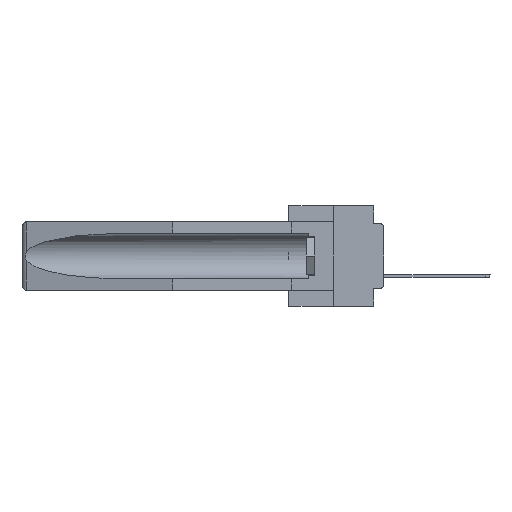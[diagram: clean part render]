
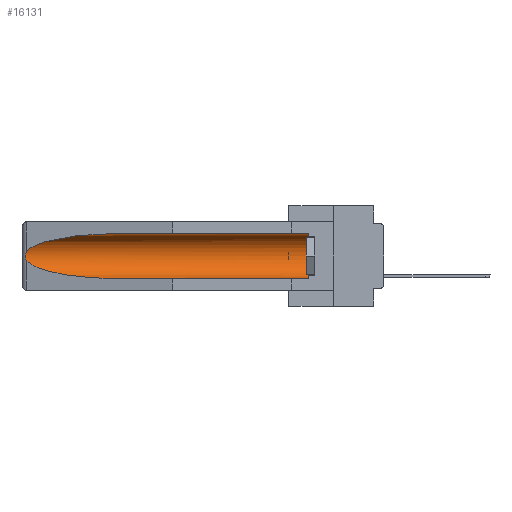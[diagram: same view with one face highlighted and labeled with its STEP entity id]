
A CAD part, left-side view. The second image highlights one B-rep face of the part: STEP entity #16131.
In plain terms, the highlighted cylindrical face has radius 2.857 mm (diameter 5.715 mm), a partial arc.
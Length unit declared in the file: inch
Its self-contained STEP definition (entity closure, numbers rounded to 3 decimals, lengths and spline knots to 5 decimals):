
#468 = CARTESIAN_POINT ( 'NONE',  ( 0.26537, 1.52718, -0.14972 ) ) ;
#720 = EDGE_CURVE ( 'NONE', #23461, #37545, #6997, .T. ) ;
#1621 = CARTESIAN_POINT ( 'NONE',  ( 0.2673, 1.53269, -0.17917 ) ) ;
#3611 = CIRCLE ( 'NONE', #32259, 0.1125 ) ;
#3714 = CYLINDRICAL_SURFACE ( 'NONE', #25135, 0.1125 ) ;
#4158 = FACE_OUTER_BOUND ( 'NONE', #36566, .T. ) ;
#4191 = CARTESIAN_POINT ( 'NONE',  ( 0.2675, 1.53308, -0.16763 ) ) ;
#4538 = VECTOR ( 'NONE', #9666, 39.37008 ) ;
#4730 = CARTESIAN_POINT ( 'NONE',  ( 0.26597, 1.5296, -0.19026 ) ) ;
#4777 = CARTESIAN_POINT ( 'NONE',  ( 0.155, -0.30754, -0.1715 ) ) ;
#5171 = EDGE_CURVE ( 'NONE', #23461, #20701, #3611, .T. ) ;
#5293 = DIRECTION ( 'NONE',  ( 0., 1., 0. ) ) ;
#6997 = LINE ( 'NONE', #7758, #8946 ) ;
#7758 = CARTESIAN_POINT ( 'NONE',  ( 0.155, -0.30754, -0.284 ) ) ;
#8514 = DIRECTION ( 'NONE',  ( 0., 0., 1. ) ) ;
#8946 = VECTOR ( 'NONE', #29276, 39.37008 ) ;
#8995 = DIRECTION ( 'NONE',  ( 0., 0., 1. ) ) ;
#9666 = DIRECTION ( 'NONE',  ( 0., 1., 0. ) ) ;
#11897 = EDGE_CURVE ( 'NONE', #32058, #24717, #37522, .T. ) ;
#11939 = CARTESIAN_POINT ( 'NONE',  ( 0.25451, 1.48313, -0.09465 ) ) ;
#12513 = VERTEX_POINT ( 'NONE', #27570 ) ;
#13298 = CARTESIAN_POINT ( 'NONE',  ( 0.26654, 1.53092, -0.15636 ) ) ;
#13831 = CARTESIAN_POINT ( 'NONE',  ( 0.2673, 1.5327, -0.16383 ) ) ;
#15137 = ORIENTED_EDGE ( 'NONE', *, *, #34715, .T. ) ;
#15309 = CARTESIAN_POINT ( 'NONE',  ( 0.155, -0.30754, -0.059 ) ) ;
#16131 = ADVANCED_FACE ( 'NONE', ( #4158 ), #3714, .F. ) ;
#16819 = CARTESIAN_POINT ( 'NONE',  ( 0.26537, 1.52718, -0.14972 ) ) ;
#18142 = CARTESIAN_POINT ( 'NONE',  ( 0.26537, 1.52718, -0.14972 ) ) ;
#18257 = CARTESIAN_POINT ( 'NONE',  ( 0.155, 0.126, -0.284 ) ) ;
#18539 = CARTESIAN_POINT ( 'NONE',  ( 0.25451, 1.48313, -0.24835 ) ) ;
#18701 = ORIENTED_EDGE ( 'NONE', *, *, #11897, .T. ) ;
#19515 = CARTESIAN_POINT ( 'NONE',  ( 0.26597, 1.52961, -0.15275 ) ) ;
#20701 = VERTEX_POINT ( 'NONE', #30123 ) ;
#23461 = VERTEX_POINT ( 'NONE', #18257 ) ;
#23571 = CARTESIAN_POINT ( 'NONE',  ( 0.155, 1.07973, -0.284 ) ) ;
#24481 = DIRECTION ( 'NONE',  ( 0., -1., 0. ) ) ;
#24717 = VERTEX_POINT ( 'NONE', #468 ) ;
#25042 = CARTESIAN_POINT ( 'NONE',  ( 0.26537, 1.52718, -0.19328 ) ) ;
#25135 = AXIS2_PLACEMENT_3D ( 'NONE', #4777, #5293, #8514 ) ;
#26280 = CARTESIAN_POINT ( 'NONE',  ( 0.26537, 1.52718, -0.19328 ) ) ;
#27570 = CARTESIAN_POINT ( 'NONE',  ( 0.26537, 1.52718, -0.19328 ) ) ;
#27589 = CARTESIAN_POINT ( 'NONE',  ( 0.21114, 1.30732, -0.284 ) ) ;
#29276 = DIRECTION ( 'NONE',  ( 0., 1., 0. ) ) ;
#30123 = CARTESIAN_POINT ( 'NONE',  ( 0.155, 0.126, -0.059 ) ) ;
#30777 = ORIENTED_EDGE ( 'NONE', *, *, #5171, .T. ) ;
#31809 = ORIENTED_EDGE ( 'NONE', *, *, #34392, .T. ) ;
#32015 = CARTESIAN_POINT ( 'NONE',  ( 0.26655, 1.53094, -0.18657 ) ) ;
#32058 = VERTEX_POINT ( 'NONE', #32993 ) ;
#32115 =( BOUNDED_CURVE ( )  B_SPLINE_CURVE ( 3, ( #25042, #18539, #27589, #36830 ),
 .UNSPECIFIED., .F., .T. ) 
 B_SPLINE_CURVE_WITH_KNOTS ( ( 4, 4 ),
 ( 0.1948, 1.5708 ),
 .UNSPECIFIED. ) 
 CURVE ( )  GEOMETRIC_REPRESENTATION_ITEM ( )  RATIONAL_B_SPLINE_CURVE ( ( 1., 0.848, 0.848, 1. ) ) 
 REPRESENTATION_ITEM ( '' )  );
#32259 = AXIS2_PLACEMENT_3D ( 'NONE', #39631, #24481, #8995 ) ;
#32327 = ORIENTED_EDGE ( 'NONE', *, *, #720, .F. ) ;
#32993 = CARTESIAN_POINT ( 'NONE',  ( 0.155, 1.07973, -0.059 ) ) ;
#33305 = EDGE_CURVE ( 'NONE', #20701, #32058, #38188, .T. ) ;
#33340 = B_SPLINE_CURVE_WITH_KNOTS ( 'NONE', 3,
 ( #16819, #19515, #13298, #13831, #4191, #38449, #1621, #32015, #4730, #26280 ),
 .UNSPECIFIED., .F., .F.,
 ( 4, 2, 2, 2, 4 ),
 ( 0., 0.00029, 0.00058, 0.00087, 0.00117 ),
 .UNSPECIFIED. ) ;
#34392 = EDGE_CURVE ( 'NONE', #24717, #12513, #33340, .T. ) ;
#34715 = EDGE_CURVE ( 'NONE', #12513, #37545, #32115, .T. ) ;
#35775 = ORIENTED_EDGE ( 'NONE', *, *, #33305, .T. ) ;
#36566 = EDGE_LOOP ( 'NONE', ( #18701, #31809, #15137, #32327, #30777, #35775 ) ) ;
#36568 = CARTESIAN_POINT ( 'NONE',  ( 0.155, 1.07973, -0.059 ) ) ;
#36830 = CARTESIAN_POINT ( 'NONE',  ( 0.155, 1.07973, -0.284 ) ) ;
#37522 =( BOUNDED_CURVE ( )  B_SPLINE_CURVE ( 3, ( #36568, #39518, #11939, #18142 ),
 .UNSPECIFIED., .F., .T. ) 
 B_SPLINE_CURVE_WITH_KNOTS ( ( 4, 4 ),
 ( 4.71239, 6.08839 ),
 .UNSPECIFIED. ) 
 CURVE ( )  GEOMETRIC_REPRESENTATION_ITEM ( )  RATIONAL_B_SPLINE_CURVE ( ( 1., 0.848, 0.848, 1. ) ) 
 REPRESENTATION_ITEM ( '' )  );
#37545 = VERTEX_POINT ( 'NONE', #23571 ) ;
#38188 = LINE ( 'NONE', #15309, #4538 ) ;
#38449 = CARTESIAN_POINT ( 'NONE',  ( 0.2675, 1.53308, -0.17534 ) ) ;
#39518 = CARTESIAN_POINT ( 'NONE',  ( 0.21114, 1.30732, -0.059 ) ) ;
#39631 = CARTESIAN_POINT ( 'NONE',  ( 0.155, 0.126, -0.1715 ) ) ;
